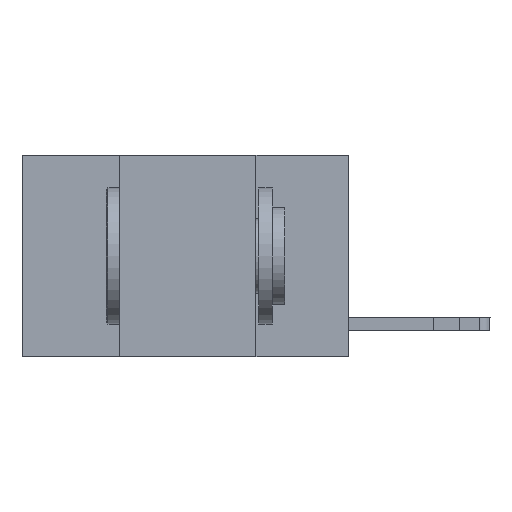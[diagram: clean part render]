
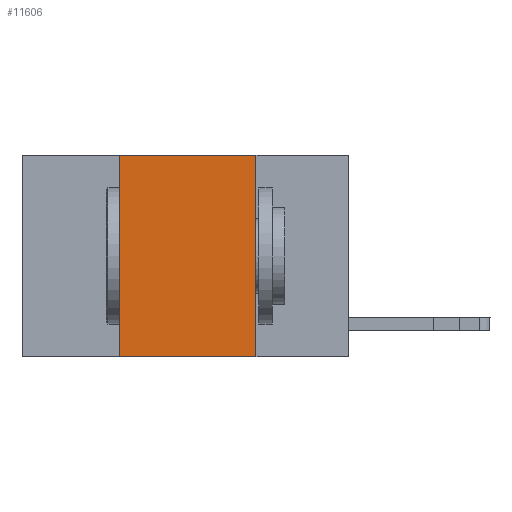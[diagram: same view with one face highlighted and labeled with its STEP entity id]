
A CAD part, left-side view. The second image highlights one B-rep face of the part: STEP entity #11606.
In plain terms, the highlighted planar face has unit normal (-1, 0, 0).
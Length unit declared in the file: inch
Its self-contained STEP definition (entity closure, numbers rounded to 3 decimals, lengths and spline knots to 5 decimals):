
#169 = DIRECTION ( 'NONE',  ( 0., -1., 0. ) ) ;
#336 = EDGE_CURVE ( 'NONE', #10084, #19910, #17287, .T. ) ;
#676 = CARTESIAN_POINT ( 'NONE',  ( 0., 0.42, -0.37 ) ) ;
#1208 = DIRECTION ( 'NONE',  ( 0., 0., -1. ) ) ;
#1414 = VERTEX_POINT ( 'NONE', #676 ) ;
#2847 = FACE_OUTER_BOUND ( 'NONE', #12419, .T. ) ;
#3205 = DIRECTION ( 'NONE',  ( 0., 0., 1. ) ) ;
#3648 = CARTESIAN_POINT ( 'NONE',  ( 0., 0.6, 0. ) ) ;
#4821 = CARTESIAN_POINT ( 'NONE',  ( 0., 0.17, 0. ) ) ;
#6255 = DIRECTION ( 'NONE',  ( 1., 0., 0. ) ) ;
#7334 = CARTESIAN_POINT ( 'NONE',  ( 0., 0.17, -0.37 ) ) ;
#7653 = VECTOR ( 'NONE', #19383, 39.37008 ) ;
#7885 = DIRECTION ( 'NONE',  ( 0., 0., -1. ) ) ;
#7892 = VERTEX_POINT ( 'NONE', #14904 ) ;
#9175 = PLANE ( 'NONE',  #10219 ) ;
#9446 = CARTESIAN_POINT ( 'NONE',  ( 0., 0.17, 0. ) ) ;
#10084 = VERTEX_POINT ( 'NONE', #4821 ) ;
#10219 = AXIS2_PLACEMENT_3D ( 'NONE', #18577, #6255, #1208 ) ;
#11095 = CARTESIAN_POINT ( 'NONE',  ( 0., 0.6, -0.37 ) ) ;
#11606 = ADVANCED_FACE ( 'NONE', ( #2847 ), #9175, .F. ) ;
#11839 = ORIENTED_EDGE ( 'NONE', *, *, #17730, .F. ) ;
#11940 = ORIENTED_EDGE ( 'NONE', *, *, #14399, .T. ) ;
#12419 = EDGE_LOOP ( 'NONE', ( #16645, #11839, #16112, #11940 ) ) ;
#12698 = LINE ( 'NONE', #13974, #15276 ) ;
#13047 = LINE ( 'NONE', #3648, #7653 ) ;
#13974 = CARTESIAN_POINT ( 'NONE',  ( 0., 0.42, 0. ) ) ;
#14399 = EDGE_CURVE ( 'NONE', #1414, #19910, #17194, .T. ) ;
#14904 = CARTESIAN_POINT ( 'NONE',  ( 0., 0.42, 0. ) ) ;
#15276 = VECTOR ( 'NONE', #3205, 39.37008 ) ;
#16112 = ORIENTED_EDGE ( 'NONE', *, *, #19661, .F. ) ;
#16364 = VECTOR ( 'NONE', #7885, 39.37008 ) ;
#16645 = ORIENTED_EDGE ( 'NONE', *, *, #336, .F. ) ;
#17033 = VECTOR ( 'NONE', #169, 39.37008 ) ;
#17194 = LINE ( 'NONE', #11095, #17033 ) ;
#17287 = LINE ( 'NONE', #9446, #16364 ) ;
#17730 = EDGE_CURVE ( 'NONE', #7892, #10084, #13047, .T. ) ;
#18577 = CARTESIAN_POINT ( 'NONE',  ( 0., 0.6, 0. ) ) ;
#19383 = DIRECTION ( 'NONE',  ( 0., -1., 0. ) ) ;
#19661 = EDGE_CURVE ( 'NONE', #1414, #7892, #12698, .T. ) ;
#19910 = VERTEX_POINT ( 'NONE', #7334 ) ;
